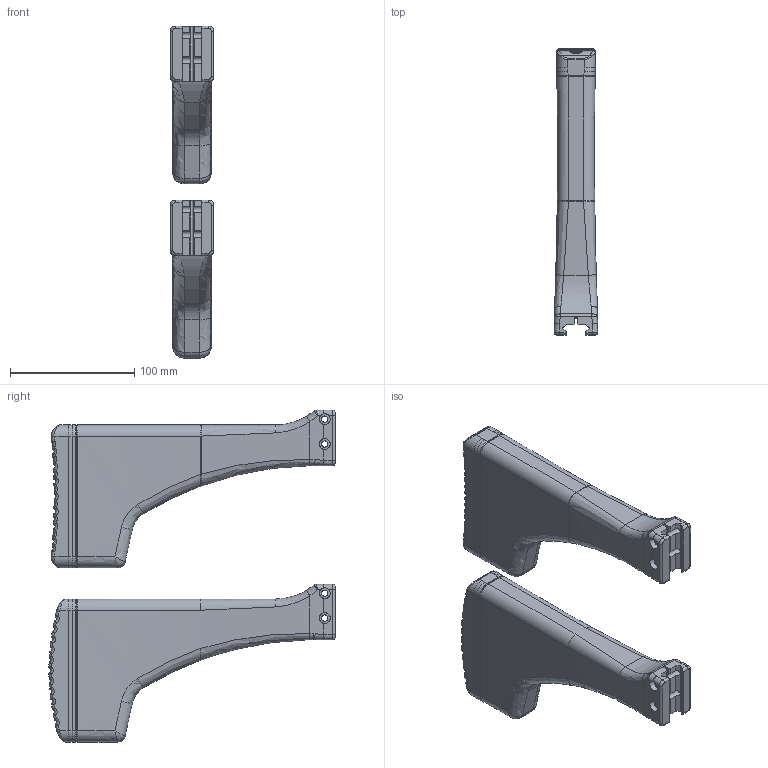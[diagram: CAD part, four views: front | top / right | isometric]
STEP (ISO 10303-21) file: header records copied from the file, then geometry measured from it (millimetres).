
FILE_DESCRIPTION(/* description */ (''),/* implementation_level */ '2;1');
FILE_NAME(/* name */ 'Final Concepts.step',/* time_stamp */ '2021-07-28T09:02:25-04:00',/* author */ (''),/* organization */ (''),/* preprocessor_version */ 'ST-DEVELOPER v18.1',/* originating_system */ 'Autodesk Translation Framework v10.9.0.1377',/* authorisation */ '');
FILE_SCHEMA (('AUTOMOTIVE_DESIGN { 1 0 10303 214 3 1 1 }'));
Length unit declared in the file: millimetre
Products named in the file (1): Final Concept
Bounding box: 35 x 230.16 x 267 mm (x, y, z)
Volume: 600667.2 mm3; surface area: 157065.1 mm2
Topology: 5 solids, 6 shells, 970 faces, 2377 edges, 1305 vertices
Faces by surface type: bspline 335, cylinder 242, plane 204, torus 170, cone 19
Full cylindrical faces by diameter (mm): 4 x8, 5.1 x8, 6.7 x14, 8 x4, 8.75 x4
Entity records: 42835 total; most frequent: CARTESIAN_POINT 22682, ORIENTED_EDGE 4494, DIRECTION 3651, EDGE_CURVE 2247, AXIS2_PLACEMENT_3D 1473, VERTEX_POINT 1305, EDGE_LOOP 1018, FACE_OUTER_BOUND 970
